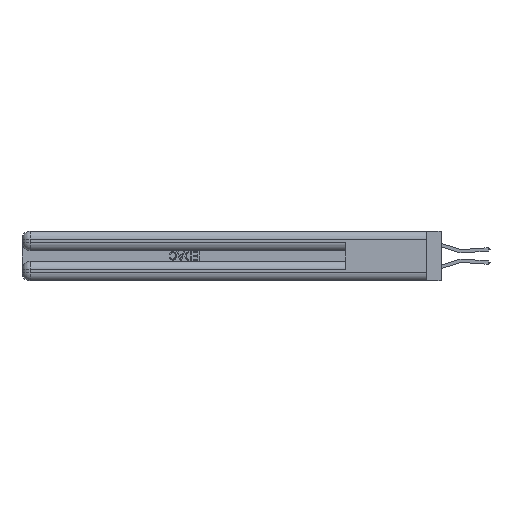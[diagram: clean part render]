
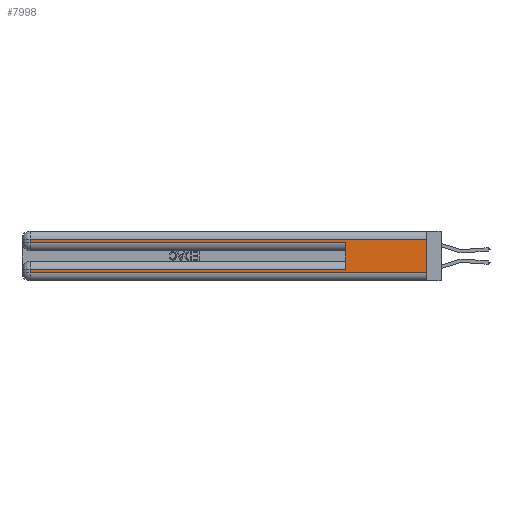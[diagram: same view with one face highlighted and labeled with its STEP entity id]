
A CAD part, left-side view. The second image highlights one B-rep face of the part: STEP entity #7998.
In plain terms, the highlighted planar face has unit normal (-1, 0, 0).
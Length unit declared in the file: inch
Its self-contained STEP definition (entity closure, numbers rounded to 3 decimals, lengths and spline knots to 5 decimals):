
#14 = FACE_OUTER_BOUND ( 'NONE', #22042, .T. ) ;
#296 = VERTEX_POINT ( 'NONE', #33725 ) ;
#865 = EDGE_CURVE ( 'NONE', #34231, #14736, #35062, .T. ) ;
#2442 = VECTOR ( 'NONE', #20969, 39.37008 ) ;
#3606 = VECTOR ( 'NONE', #34747, 39.37008 ) ;
#7998 = ADVANCED_FACE ( 'NONE', ( #14 ), #21550, .F. ) ;
#8615 = CARTESIAN_POINT ( 'NONE',  ( 0., 0., 0.31 ) ) ;
#9510 = VERTEX_POINT ( 'NONE', #20304 ) ;
#10449 = EDGE_CURVE ( 'NONE', #14792, #296, #15684, .T. ) ;
#11238 = ORIENTED_EDGE ( 'NONE', *, *, #11500, .T. ) ;
#11312 = VERTEX_POINT ( 'NONE', #12415 ) ;
#11500 = EDGE_CURVE ( 'NONE', #14534, #34231, #18933, .T. ) ;
#12387 = DIRECTION ( 'NONE',  ( 0., 1., 0. ) ) ;
#12415 = CARTESIAN_POINT ( 'NONE',  ( 0., 0.6, 0.085 ) ) ;
#12444 = CARTESIAN_POINT ( 'NONE',  ( 0., 0., 0.37 ) ) ;
#13909 = ORIENTED_EDGE ( 'NONE', *, *, #15803, .F. ) ;
#14534 = VERTEX_POINT ( 'NONE', #8615 ) ;
#14684 = ORIENTED_EDGE ( 'NONE', *, *, #22045, .T. ) ;
#14736 = VERTEX_POINT ( 'NONE', #27948 ) ;
#14792 = VERTEX_POINT ( 'NONE', #37041 ) ;
#15521 = DIRECTION ( 'NONE',  ( 0., 0., -1. ) ) ;
#15684 = LINE ( 'NONE', #22530, #31967 ) ;
#15803 = EDGE_CURVE ( 'NONE', #14534, #296, #26910, .T. ) ;
#17042 = ORIENTED_EDGE ( 'NONE', *, *, #10449, .T. ) ;
#17267 = EDGE_CURVE ( 'NONE', #11312, #23501, #24890, .T. ) ;
#17864 = VECTOR ( 'NONE', #22379, 39.37008 ) ;
#18092 = DIRECTION ( 'NONE',  ( 0., 0., -1. ) ) ;
#18933 = LINE ( 'NONE', #22449, #3606 ) ;
#19920 = CARTESIAN_POINT ( 'NONE',  ( 0., 0.6, 0.145 ) ) ;
#20304 = CARTESIAN_POINT ( 'NONE',  ( 0., 0.6, 0.285 ) ) ;
#20562 = LINE ( 'NONE', #19920, #25882 ) ;
#20607 = ORIENTED_EDGE ( 'NONE', *, *, #36431, .F. ) ;
#20969 = DIRECTION ( 'NONE',  ( 0., 0., -1. ) ) ;
#21550 = PLANE ( 'NONE',  #26390 ) ;
#21745 = ORIENTED_EDGE ( 'NONE', *, *, #33760, .T. ) ;
#22042 = EDGE_LOOP ( 'NONE', ( #13909, #11238, #28280, #14684, #20607, #39499, #21745, #17042 ) ) ;
#22045 = EDGE_CURVE ( 'NONE', #14736, #9510, #24125, .T. ) ;
#22379 = DIRECTION ( 'NONE',  ( 0., -1., 0. ) ) ;
#22449 = CARTESIAN_POINT ( 'NONE',  ( 0., 0., 0.31 ) ) ;
#22530 = CARTESIAN_POINT ( 'NONE',  ( 0., 0., 0.06 ) ) ;
#23501 = VERTEX_POINT ( 'NONE', #29224 ) ;
#23620 = LINE ( 'NONE', #33368, #38899 ) ;
#24125 = LINE ( 'NONE', #37608, #17864 ) ;
#24890 = LINE ( 'NONE', #36861, #33952 ) ;
#25628 = DIRECTION ( 'NONE',  ( 0., -1., 0. ) ) ;
#25882 = VECTOR ( 'NONE', #38243, 39.37008 ) ;
#26390 = AXIS2_PLACEMENT_3D ( 'NONE', #12444, #33860, #15521 ) ;
#26569 = CARTESIAN_POINT ( 'NONE',  ( 0., 0., 0.37 ) ) ;
#26910 = LINE ( 'NONE', #26569, #27875 ) ;
#27875 = VECTOR ( 'NONE', #38683, 39.37008 ) ;
#27948 = CARTESIAN_POINT ( 'NONE',  ( 0., 2.94, 0.285 ) ) ;
#28280 = ORIENTED_EDGE ( 'NONE', *, *, #865, .T. ) ;
#29224 = CARTESIAN_POINT ( 'NONE',  ( 0., 2.94, 0.085 ) ) ;
#30078 = CARTESIAN_POINT ( 'NONE',  ( 0., 2.94, 0.37 ) ) ;
#31967 = VECTOR ( 'NONE', #25628, 39.37008 ) ;
#32824 = CARTESIAN_POINT ( 'NONE',  ( 0., 2.94, 0.31 ) ) ;
#33368 = CARTESIAN_POINT ( 'NONE',  ( 0., 2.94, 0.37 ) ) ;
#33725 = CARTESIAN_POINT ( 'NONE',  ( 0., 0., 0.06 ) ) ;
#33760 = EDGE_CURVE ( 'NONE', #23501, #14792, #23620, .T. ) ;
#33860 = DIRECTION ( 'NONE',  ( 1., 0., 0. ) ) ;
#33952 = VECTOR ( 'NONE', #12387, 39.37008 ) ;
#34231 = VERTEX_POINT ( 'NONE', #32824 ) ;
#34747 = DIRECTION ( 'NONE',  ( 0., 1., 0. ) ) ;
#35062 = LINE ( 'NONE', #30078, #2442 ) ;
#36431 = EDGE_CURVE ( 'NONE', #11312, #9510, #20562, .T. ) ;
#36861 = CARTESIAN_POINT ( 'NONE',  ( 0., 0., 0.085 ) ) ;
#37041 = CARTESIAN_POINT ( 'NONE',  ( 0., 2.94, 0.06 ) ) ;
#37608 = CARTESIAN_POINT ( 'NONE',  ( 0., 0., 0.285 ) ) ;
#38243 = DIRECTION ( 'NONE',  ( 0., 0., 1. ) ) ;
#38683 = DIRECTION ( 'NONE',  ( 0., 0., -1. ) ) ;
#38899 = VECTOR ( 'NONE', #18092, 39.37008 ) ;
#39499 = ORIENTED_EDGE ( 'NONE', *, *, #17267, .T. ) ;
